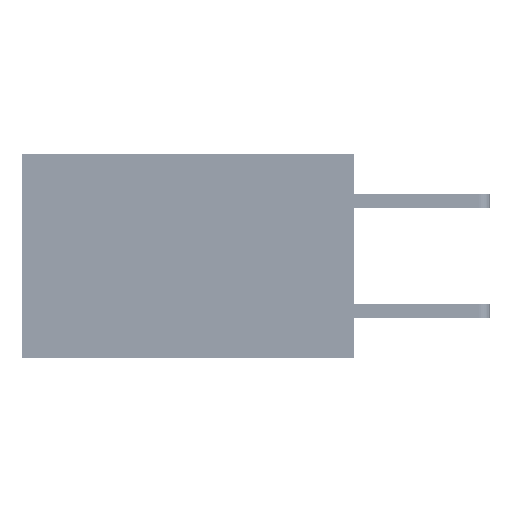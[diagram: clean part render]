
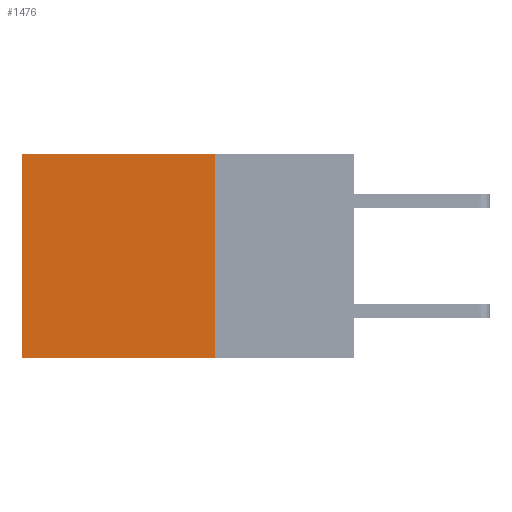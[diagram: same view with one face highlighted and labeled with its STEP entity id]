
A CAD part, left-side view. The second image highlights one B-rep face of the part: STEP entity #1476.
In plain terms, the highlighted planar face has unit normal (-1, 0, 0).
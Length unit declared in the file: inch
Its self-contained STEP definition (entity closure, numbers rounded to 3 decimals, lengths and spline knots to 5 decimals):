
#381 = DIRECTION ( 'NONE',  ( 0., 1., 0. ) ) ;
#1476 = ADVANCED_FACE ( 'NONE', ( #26913 ), #27551, .F. ) ;
#3780 = VECTOR ( 'NONE', #381, 39.37008 ) ;
#10926 = CARTESIAN_POINT ( 'NONE',  ( 0.2875, 0.25, -0.37 ) ) ;
#10968 = DIRECTION ( 'NONE',  ( 1., 0., 0. ) ) ;
#11380 = CARTESIAN_POINT ( 'NONE',  ( 0.2875, 0.25, 0. ) ) ;
#11617 = EDGE_CURVE ( 'NONE', #15212, #21600, #33758, .T. ) ;
#15212 = VERTEX_POINT ( 'NONE', #10926 ) ;
#15637 = LINE ( 'NONE', #18907, #28033 ) ;
#15855 = CARTESIAN_POINT ( 'NONE',  ( 0.2875, 0.6, 0. ) ) ;
#18383 = EDGE_CURVE ( 'NONE', #18423, #15212, #31010, .T. ) ;
#18423 = VERTEX_POINT ( 'NONE', #21623 ) ;
#18907 = CARTESIAN_POINT ( 'NONE',  ( 0.2875, 0.25, 0. ) ) ;
#20450 = EDGE_CURVE ( 'NONE', #18423, #36639, #15637, .T. ) ;
#21195 = DIRECTION ( 'NONE',  ( 0., 0., -1. ) ) ;
#21535 = ORIENTED_EDGE ( 'NONE', *, *, #42284, .T. ) ;
#21600 = VERTEX_POINT ( 'NONE', #25015 ) ;
#21623 = CARTESIAN_POINT ( 'NONE',  ( 0.2875, 0.25, 0. ) ) ;
#24077 = CARTESIAN_POINT ( 'NONE',  ( 0.2875, 0.6, 0. ) ) ;
#24272 = DIRECTION ( 'NONE',  ( 0., 0., -1. ) ) ;
#25015 = CARTESIAN_POINT ( 'NONE',  ( 0.2875, 0.6, -0.37 ) ) ;
#26102 = LINE ( 'NONE', #15855, #28085 ) ;
#26913 = FACE_OUTER_BOUND ( 'NONE', #39210, .T. ) ;
#27551 = PLANE ( 'NONE',  #30498 ) ;
#28033 = VECTOR ( 'NONE', #35458, 39.37008 ) ;
#28085 = VECTOR ( 'NONE', #29157, 39.37008 ) ;
#29157 = DIRECTION ( 'NONE',  ( 0., 0., -1. ) ) ;
#30498 = AXIS2_PLACEMENT_3D ( 'NONE', #40839, #10968, #24272 ) ;
#31010 = LINE ( 'NONE', #11380, #38523 ) ;
#33758 = LINE ( 'NONE', #36591, #3780 ) ;
#35458 = DIRECTION ( 'NONE',  ( 0., 1., 0. ) ) ;
#35737 = ORIENTED_EDGE ( 'NONE', *, *, #11617, .F. ) ;
#35876 = ORIENTED_EDGE ( 'NONE', *, *, #20450, .T. ) ;
#36591 = CARTESIAN_POINT ( 'NONE',  ( 0.2875, 0.25, -0.37 ) ) ;
#36639 = VERTEX_POINT ( 'NONE', #24077 ) ;
#38523 = VECTOR ( 'NONE', #21195, 39.37008 ) ;
#39210 = EDGE_LOOP ( 'NONE', ( #21535, #35737, #42117, #35876 ) ) ;
#40839 = CARTESIAN_POINT ( 'NONE',  ( 0.2875, 0.25, 0. ) ) ;
#42117 = ORIENTED_EDGE ( 'NONE', *, *, #18383, .F. ) ;
#42284 = EDGE_CURVE ( 'NONE', #36639, #21600, #26102, .T. ) ;
